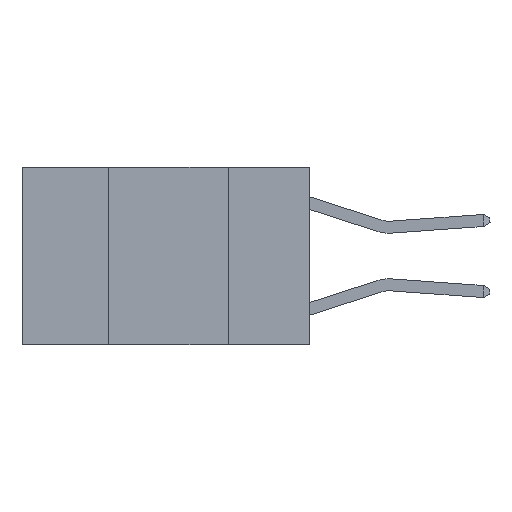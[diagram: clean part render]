
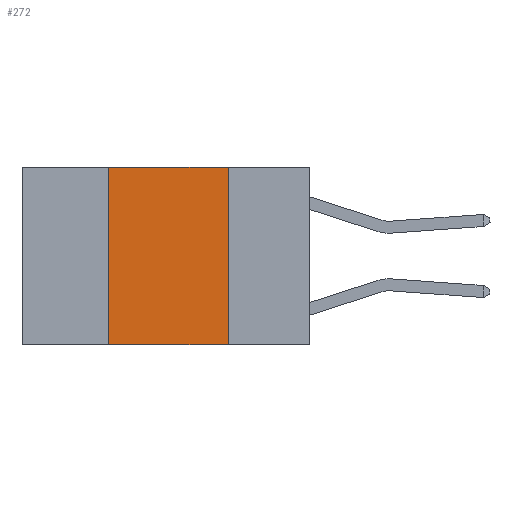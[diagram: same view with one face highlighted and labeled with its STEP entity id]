
A CAD part, left-side view. The second image highlights one B-rep face of the part: STEP entity #272.
In plain terms, the highlighted planar face has unit normal (-1, 0, 0).
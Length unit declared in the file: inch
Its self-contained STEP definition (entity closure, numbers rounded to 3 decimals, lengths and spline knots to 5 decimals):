
#264 = EDGE_LOOP ( 'NONE', ( #8755, #2689, #10010, #2114 ) ) ;
#272 = ADVANCED_FACE ( 'NONE', ( #1047 ), #2527, .F. ) ;
#503 = EDGE_CURVE ( 'NONE', #536, #8179, #1518, .T. ) ;
#536 = VERTEX_POINT ( 'NONE', #6675 ) ;
#670 = VECTOR ( 'NONE', #10436, 39.37008 ) ;
#767 = CARTESIAN_POINT ( 'NONE',  ( 0., 0.17, 0. ) ) ;
#1047 = FACE_OUTER_BOUND ( 'NONE', #264, .T. ) ;
#1431 = CARTESIAN_POINT ( 'NONE',  ( 0., 0.6, 0. ) ) ;
#1479 = VECTOR ( 'NONE', #3843, 39.37008 ) ;
#1518 = LINE ( 'NONE', #1679, #1479 ) ;
#1679 = CARTESIAN_POINT ( 'NONE',  ( 0., 0.6, -0.37 ) ) ;
#2114 = ORIENTED_EDGE ( 'NONE', *, *, #503, .T. ) ;
#2135 = CARTESIAN_POINT ( 'NONE',  ( 0., 0.17, 0. ) ) ;
#2527 = PLANE ( 'NONE',  #9104 ) ;
#2658 = CARTESIAN_POINT ( 'NONE',  ( 0., 0.42, 0. ) ) ;
#2671 = DIRECTION ( 'NONE',  ( 1., 0., 0. ) ) ;
#2689 = ORIENTED_EDGE ( 'NONE', *, *, #3158, .F. ) ;
#2846 = LINE ( 'NONE', #1431, #3070 ) ;
#2951 = DIRECTION ( 'NONE',  ( 0., -1., 0. ) ) ;
#2959 = EDGE_CURVE ( 'NONE', #536, #7059, #7518, .T. ) ;
#3070 = VECTOR ( 'NONE', #2951, 39.37008 ) ;
#3158 = EDGE_CURVE ( 'NONE', #7059, #9935, #2846, .T. ) ;
#3506 = DIRECTION ( 'NONE',  ( 0., 0., 1. ) ) ;
#3843 = DIRECTION ( 'NONE',  ( 0., -1., 0. ) ) ;
#4096 = LINE ( 'NONE', #767, #670 ) ;
#4290 = CARTESIAN_POINT ( 'NONE',  ( 0., 0.6, 0. ) ) ;
#4781 = VECTOR ( 'NONE', #3506, 39.37008 ) ;
#6675 = CARTESIAN_POINT ( 'NONE',  ( 0., 0.42, -0.37 ) ) ;
#7059 = VERTEX_POINT ( 'NONE', #10315 ) ;
#7454 = EDGE_CURVE ( 'NONE', #9935, #8179, #4096, .T. ) ;
#7518 = LINE ( 'NONE', #2658, #4781 ) ;
#7912 = CARTESIAN_POINT ( 'NONE',  ( 0., 0.17, -0.37 ) ) ;
#8179 = VERTEX_POINT ( 'NONE', #7912 ) ;
#8334 = DIRECTION ( 'NONE',  ( 0., 0., -1. ) ) ;
#8755 = ORIENTED_EDGE ( 'NONE', *, *, #7454, .F. ) ;
#9104 = AXIS2_PLACEMENT_3D ( 'NONE', #4290, #2671, #8334 ) ;
#9935 = VERTEX_POINT ( 'NONE', #2135 ) ;
#10010 = ORIENTED_EDGE ( 'NONE', *, *, #2959, .F. ) ;
#10315 = CARTESIAN_POINT ( 'NONE',  ( 0., 0.42, 0. ) ) ;
#10436 = DIRECTION ( 'NONE',  ( 0., 0., -1. ) ) ;
